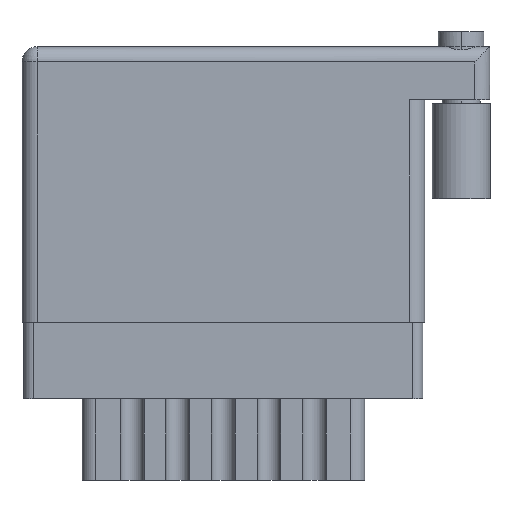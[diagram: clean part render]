
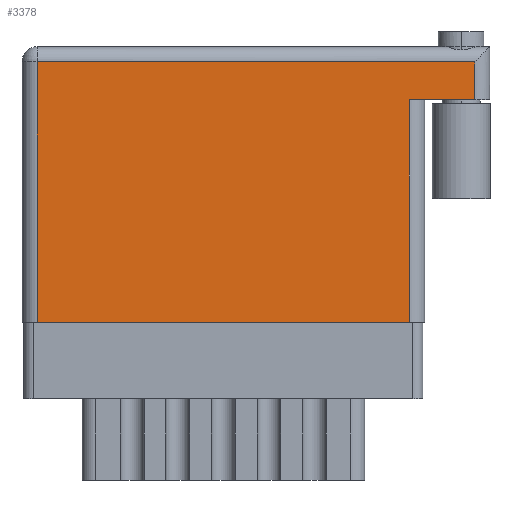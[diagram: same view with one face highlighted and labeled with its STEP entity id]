
A CAD part, front view. The second image highlights one B-rep face of the part: STEP entity #3378.
In plain terms, the highlighted face is planar.
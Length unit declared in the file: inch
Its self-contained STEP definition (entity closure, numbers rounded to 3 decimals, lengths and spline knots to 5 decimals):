
#1574 = EDGE_LOOP ( 'NONE', ( #12716, #12963, #16127, #19756, #15778, #14012 ) ) ;
#1849 = VECTOR ( 'NONE', #7203, 39.37008 ) ;
#3378 = ADVANCED_FACE ( 'NONE', ( #21117 ), #6192, .F. ) ;
#3506 = VERTEX_POINT ( 'NONE', #10422 ) ;
#3740 = LINE ( 'NONE', #10255, #1849 ) ;
#4039 = DIRECTION ( 'NONE',  ( -1., 0., 0. ) ) ;
#4164 = VECTOR ( 'NONE', #15218, 39.37008 ) ;
#4477 = EDGE_CURVE ( 'NONE', #6562, #3506, #15789, .T. ) ;
#4715 = EDGE_CURVE ( 'NONE', #8778, #17078, #13182, .T. ) ;
#5352 = EDGE_CURVE ( 'NONE', #17078, #21427, #8609, .T. ) ;
#6103 = CARTESIAN_POINT ( 'NONE',  ( 1.489, 0.856, 0. ) ) ;
#6192 = PLANE ( 'NONE',  #16257 ) ;
#6562 = VERTEX_POINT ( 'NONE', #9139 ) ;
#6731 = VECTOR ( 'NONE', #8001, 39.37008 ) ;
#6844 = VECTOR ( 'NONE', #4039, 39.37008 ) ;
#7203 = DIRECTION ( 'NONE',  ( -1., 0., 0. ) ) ;
#7429 = CARTESIAN_POINT ( 'NONE',  ( 0.05, 0.856, 0. ) ) ;
#7520 = CARTESIAN_POINT ( 'NONE',  ( 0., 0., 0. ) ) ;
#8001 = DIRECTION ( 'NONE',  ( 0., -1., 0. ) ) ;
#8087 = EDGE_CURVE ( 'NONE', #3506, #20037, #8270, .T. ) ;
#8270 = LINE ( 'NONE', #18615, #11944 ) ;
#8609 = LINE ( 'NONE', #15457, #6844 ) ;
#8778 = VERTEX_POINT ( 'NONE', #21192 ) ;
#8864 = EDGE_CURVE ( 'NONE', #21427, #6562, #18346, .T. ) ;
#9139 = CARTESIAN_POINT ( 'NONE',  ( 0.05, 0., 0. ) ) ;
#10255 = CARTESIAN_POINT ( 'NONE',  ( 1.539, 0.731, 0. ) ) ;
#10422 = CARTESIAN_POINT ( 'NONE',  ( 1.275, 0., 0. ) ) ;
#11120 = CARTESIAN_POINT ( 'NONE',  ( 1.275, 0.731, 0. ) ) ;
#11622 = DIRECTION ( 'NONE',  ( 0., 0., -1. ) ) ;
#11944 = VECTOR ( 'NONE', #19826, 39.37008 ) ;
#12716 = ORIENTED_EDGE ( 'NONE', *, *, #4477, .T. ) ;
#12963 = ORIENTED_EDGE ( 'NONE', *, *, #8087, .T. ) ;
#13182 = LINE ( 'NONE', #20249, #4164 ) ;
#14012 = ORIENTED_EDGE ( 'NONE', *, *, #8864, .T. ) ;
#14688 = CARTESIAN_POINT ( 'NONE',  ( 0., 0.906, 0. ) ) ;
#15218 = DIRECTION ( 'NONE',  ( 0., 1., 0. ) ) ;
#15457 = CARTESIAN_POINT ( 'NONE',  ( 0., 0.856, 0. ) ) ;
#15778 = ORIENTED_EDGE ( 'NONE', *, *, #5352, .T. ) ;
#15789 = LINE ( 'NONE', #7520, #18780 ) ;
#16127 = ORIENTED_EDGE ( 'NONE', *, *, #20920, .F. ) ;
#16257 = AXIS2_PLACEMENT_3D ( 'NONE', #14688, #11622, #16424 ) ;
#16424 = DIRECTION ( 'NONE',  ( -1., 0., 0. ) ) ;
#17078 = VERTEX_POINT ( 'NONE', #6103 ) ;
#18242 = CARTESIAN_POINT ( 'NONE',  ( 0.05, 0., 0. ) ) ;
#18346 = LINE ( 'NONE', #18242, #6731 ) ;
#18615 = CARTESIAN_POINT ( 'NONE',  ( 1.275, 0.731, 0. ) ) ;
#18780 = VECTOR ( 'NONE', #20822, 39.37008 ) ;
#19756 = ORIENTED_EDGE ( 'NONE', *, *, #4715, .T. ) ;
#19826 = DIRECTION ( 'NONE',  ( 0., 1., 0. ) ) ;
#20037 = VERTEX_POINT ( 'NONE', #11120 ) ;
#20249 = CARTESIAN_POINT ( 'NONE',  ( 1.489, 0.906, 0. ) ) ;
#20822 = DIRECTION ( 'NONE',  ( 1., 0., 0. ) ) ;
#20920 = EDGE_CURVE ( 'NONE', #8778, #20037, #3740, .T. ) ;
#21117 = FACE_OUTER_BOUND ( 'NONE', #1574, .T. ) ;
#21192 = CARTESIAN_POINT ( 'NONE',  ( 1.489, 0.731, 0. ) ) ;
#21427 = VERTEX_POINT ( 'NONE', #7429 ) ;
